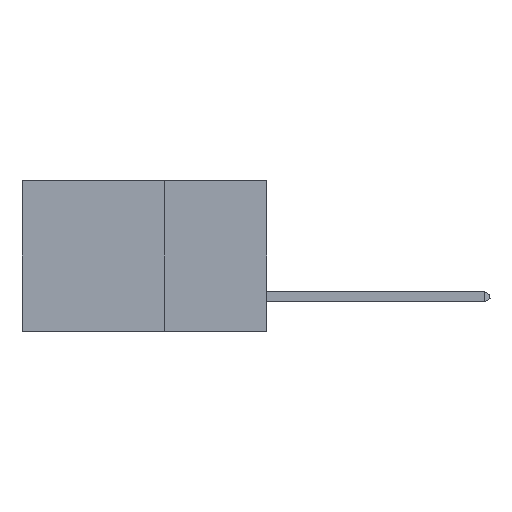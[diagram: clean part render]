
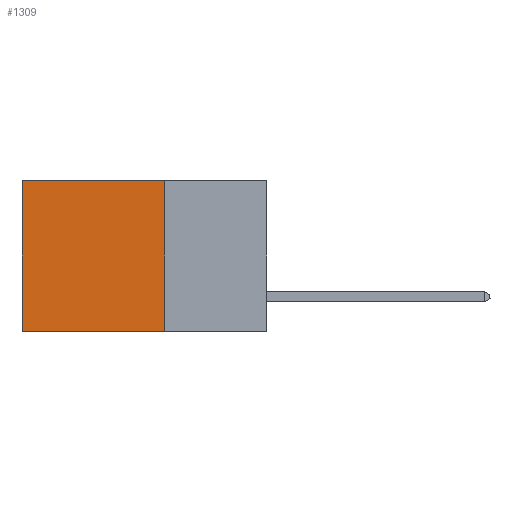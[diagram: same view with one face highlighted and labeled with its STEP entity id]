
A CAD part, left-side view. The second image highlights one B-rep face of the part: STEP entity #1309.
In plain terms, the highlighted planar face has unit normal (-1, 0, 0).
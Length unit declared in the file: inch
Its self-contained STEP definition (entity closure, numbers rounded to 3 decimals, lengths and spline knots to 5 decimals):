
#329 = ORIENTED_EDGE ( 'NONE', *, *, #13207, .F. ) ;
#492 = ORIENTED_EDGE ( 'NONE', *, *, #17454, .F. ) ;
#600 = VERTEX_POINT ( 'NONE', #18309 ) ;
#1309 = ADVANCED_FACE ( 'NONE', ( #2746 ), #13841, .F. ) ;
#2095 = LINE ( 'NONE', #16665, #4113 ) ;
#2103 = DIRECTION ( 'NONE',  ( 0., 1., 0. ) ) ;
#2746 = FACE_OUTER_BOUND ( 'NONE', #18877, .T. ) ;
#2910 = CARTESIAN_POINT ( 'NONE',  ( 0.2875, 0.25, 0. ) ) ;
#2948 = LINE ( 'NONE', #14326, #5503 ) ;
#3068 = AXIS2_PLACEMENT_3D ( 'NONE', #2910, #6743, #8579 ) ;
#4057 = VERTEX_POINT ( 'NONE', #5537 ) ;
#4113 = VECTOR ( 'NONE', #2103, 39.37008 ) ;
#4609 = CARTESIAN_POINT ( 'NONE',  ( 0.2875, 0.25, -0.37 ) ) ;
#5503 = VECTOR ( 'NONE', #12548, 39.37008 ) ;
#5537 = CARTESIAN_POINT ( 'NONE',  ( 0.2875, 0.6, 0. ) ) ;
#5882 = LINE ( 'NONE', #19268, #18197 ) ;
#6743 = DIRECTION ( 'NONE',  ( 1., 0., 0. ) ) ;
#6965 = LINE ( 'NONE', #22663, #20930 ) ;
#8579 = DIRECTION ( 'NONE',  ( 0., 0., -1. ) ) ;
#8769 = ORIENTED_EDGE ( 'NONE', *, *, #9727, .T. ) ;
#9727 = EDGE_CURVE ( 'NONE', #4057, #600, #2948, .T. ) ;
#12548 = DIRECTION ( 'NONE',  ( 0., 0., -1. ) ) ;
#13207 = EDGE_CURVE ( 'NONE', #14474, #13636, #5882, .T. ) ;
#13636 = VERTEX_POINT ( 'NONE', #4609 ) ;
#13687 = ORIENTED_EDGE ( 'NONE', *, *, #18614, .T. ) ;
#13841 = PLANE ( 'NONE',  #3068 ) ;
#14326 = CARTESIAN_POINT ( 'NONE',  ( 0.2875, 0.6, 0. ) ) ;
#14474 = VERTEX_POINT ( 'NONE', #22463 ) ;
#15459 = DIRECTION ( 'NONE',  ( 0., 0., -1. ) ) ;
#16665 = CARTESIAN_POINT ( 'NONE',  ( 0.2875, 0.25, -0.37 ) ) ;
#17454 = EDGE_CURVE ( 'NONE', #13636, #600, #2095, .T. ) ;
#18197 = VECTOR ( 'NONE', #15459, 39.37008 ) ;
#18309 = CARTESIAN_POINT ( 'NONE',  ( 0.2875, 0.6, -0.37 ) ) ;
#18614 = EDGE_CURVE ( 'NONE', #14474, #4057, #6965, .T. ) ;
#18877 = EDGE_LOOP ( 'NONE', ( #8769, #492, #329, #13687 ) ) ;
#19268 = CARTESIAN_POINT ( 'NONE',  ( 0.2875, 0.25, 0. ) ) ;
#20718 = DIRECTION ( 'NONE',  ( 0., 1., 0. ) ) ;
#20930 = VECTOR ( 'NONE', #20718, 39.37008 ) ;
#22463 = CARTESIAN_POINT ( 'NONE',  ( 0.2875, 0.25, 0. ) ) ;
#22663 = CARTESIAN_POINT ( 'NONE',  ( 0.2875, 0.25, 0. ) ) ;
